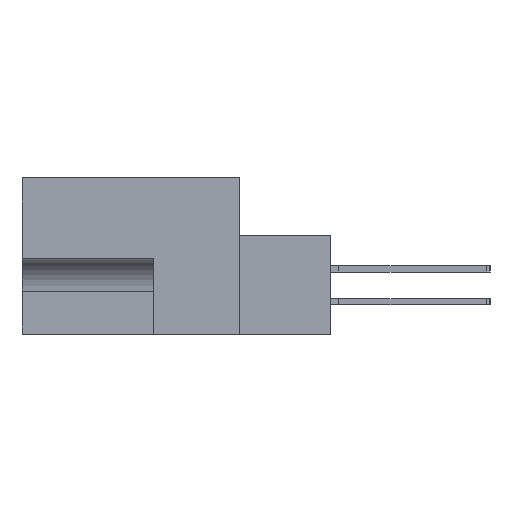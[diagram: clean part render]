
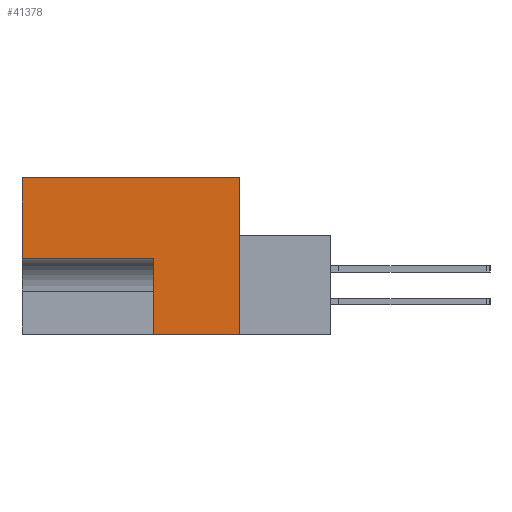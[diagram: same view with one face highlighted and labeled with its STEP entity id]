
A CAD part, left-side view. The second image highlights one B-rep face of the part: STEP entity #41378.
In plain terms, the highlighted planar face has unit normal (-1, 0, 0).
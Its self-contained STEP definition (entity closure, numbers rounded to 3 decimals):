
#125 = EDGE_CURVE ( 'NONE', #14155, #30343, #4464, .T. ) ;
#312 = VECTOR ( 'NONE', #31307, 1000. ) ;
#686 = CARTESIAN_POINT ( 'NONE',  ( 0., 0., -15.088 ) ) ;
#1641 = VERTEX_POINT ( 'NONE', #19322 ) ;
#3084 = VERTEX_POINT ( 'NONE', #38215 ) ;
#3390 = CARTESIAN_POINT ( 'NONE',  ( 0., -8.814, -15.088 ) ) ;
#4464 = LINE ( 'NONE', #3390, #28907 ) ;
#5097 = AXIS2_PLACEMENT_3D ( 'NONE', #25723, #42346, #33911 ) ;
#6270 = VECTOR ( 'NONE', #41742, 1000. ) ;
#6826 = CARTESIAN_POINT ( 'NONE',  ( 0., 0., 0. ) ) ;
#6999 = CARTESIAN_POINT ( 'NONE',  ( 0., 8.255, -15.088 ) ) ;
#8481 = ORIENTED_EDGE ( 'NONE', *, *, #19892, .F. ) ;
#9000 = CARTESIAN_POINT ( 'NONE',  ( 0., 0., 0. ) ) ;
#11535 = DIRECTION ( 'NONE',  ( 0., 1., 0. ) ) ;
#12517 = VECTOR ( 'NONE', #16121, 1000. ) ;
#12630 = CARTESIAN_POINT ( 'NONE',  ( 0., 8.255, -7.772 ) ) ;
#14155 = VERTEX_POINT ( 'NONE', #686 ) ;
#15410 = ORIENTED_EDGE ( 'NONE', *, *, #125, .F. ) ;
#16121 = DIRECTION ( 'NONE',  ( 0., 0., 1. ) ) ;
#19122 = EDGE_CURVE ( 'NONE', #1641, #22292, #47663, .T. ) ;
#19322 = CARTESIAN_POINT ( 'NONE',  ( 0., 20.955, -7.772 ) ) ;
#19892 = EDGE_CURVE ( 'NONE', #30343, #3084, #24406, .T. ) ;
#20336 = LINE ( 'NONE', #6826, #312 ) ;
#21120 = CARTESIAN_POINT ( 'NONE',  ( 0., 8.255, -15.088 ) ) ;
#22292 = VERTEX_POINT ( 'NONE', #23652 ) ;
#23075 = VECTOR ( 'NONE', #28247, 1000. ) ;
#23652 = CARTESIAN_POINT ( 'NONE',  ( 0., 20.955, 0. ) ) ;
#24210 = CARTESIAN_POINT ( 'NONE',  ( 0., 11.506, 0. ) ) ;
#24406 = LINE ( 'NONE', #21120, #6270 ) ;
#25723 = CARTESIAN_POINT ( 'NONE',  ( 0., 0., 0. ) ) ;
#25920 = EDGE_CURVE ( 'NONE', #46488, #14155, #20336, .T. ) ;
#28247 = DIRECTION ( 'NONE',  ( 0., -1., 0. ) ) ;
#28907 = VECTOR ( 'NONE', #11535, 1000. ) ;
#30343 = VERTEX_POINT ( 'NONE', #6999 ) ;
#31076 = EDGE_CURVE ( 'NONE', #22292, #46488, #34921, .T. ) ;
#31307 = DIRECTION ( 'NONE',  ( 0., 0., -1. ) ) ;
#32402 = CARTESIAN_POINT ( 'NONE',  ( 0., 20.955, -15.088 ) ) ;
#33911 = DIRECTION ( 'NONE',  ( 0., 0., -1. ) ) ;
#34093 = LINE ( 'NONE', #12630, #42270 ) ;
#34921 = LINE ( 'NONE', #24210, #23075 ) ;
#38215 = CARTESIAN_POINT ( 'NONE',  ( 0., 8.255, -7.772 ) ) ;
#38302 = ORIENTED_EDGE ( 'NONE', *, *, #40632, .F. ) ;
#38371 = FACE_OUTER_BOUND ( 'NONE', #39236, .T. ) ;
#39236 = EDGE_LOOP ( 'NONE', ( #15410, #46962, #40196, #46243, #38302, #8481 ) ) ;
#40196 = ORIENTED_EDGE ( 'NONE', *, *, #31076, .F. ) ;
#40484 = DIRECTION ( 'NONE',  ( 0., 1., 0. ) ) ;
#40632 = EDGE_CURVE ( 'NONE', #3084, #1641, #34093, .T. ) ;
#41378 = ADVANCED_FACE ( 'NONE', ( #38371 ), #45691, .F. ) ;
#41742 = DIRECTION ( 'NONE',  ( 0., 0., 1. ) ) ;
#42270 = VECTOR ( 'NONE', #40484, 1000. ) ;
#42346 = DIRECTION ( 'NONE',  ( 1., 0., 0. ) ) ;
#45691 = PLANE ( 'NONE',  #5097 ) ;
#46243 = ORIENTED_EDGE ( 'NONE', *, *, #19122, .F. ) ;
#46488 = VERTEX_POINT ( 'NONE', #9000 ) ;
#46962 = ORIENTED_EDGE ( 'NONE', *, *, #25920, .F. ) ;
#47663 = LINE ( 'NONE', #32402, #12517 ) ;
